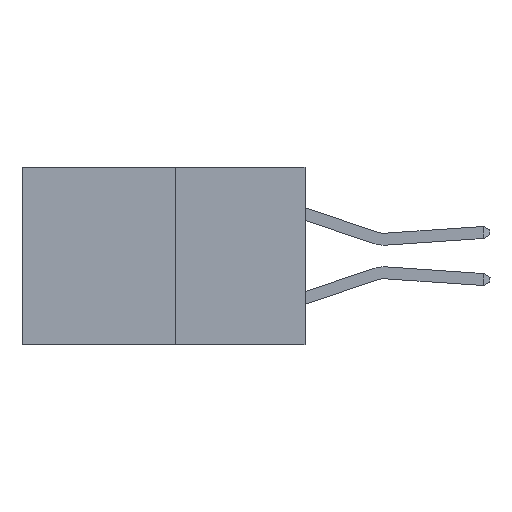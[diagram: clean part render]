
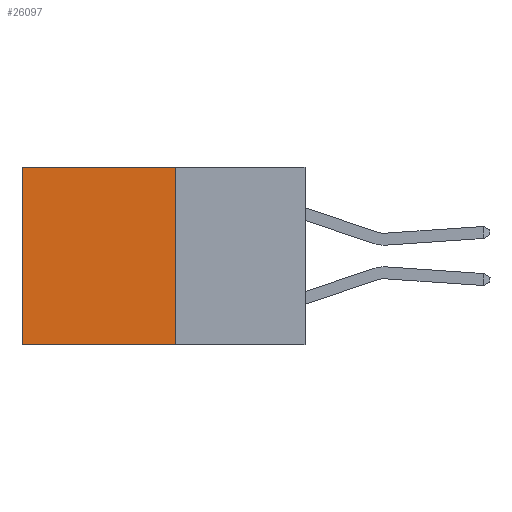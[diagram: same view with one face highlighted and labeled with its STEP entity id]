
A CAD part, left-side view. The second image highlights one B-rep face of the part: STEP entity #26097.
In plain terms, the highlighted planar face has unit normal (-1, 0, 0).
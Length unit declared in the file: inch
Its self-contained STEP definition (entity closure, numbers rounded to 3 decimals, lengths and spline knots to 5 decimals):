
#1031 = ORIENTED_EDGE ( 'NONE', *, *, #2963, .T. ) ;
#2616 = LINE ( 'NONE', #23293, #19332 ) ;
#2730 = LINE ( 'NONE', #22361, #3410 ) ;
#2963 = EDGE_CURVE ( 'NONE', #20592, #20436, #19629, .T. ) ;
#3410 = VECTOR ( 'NONE', #9292, 39.37008 ) ;
#3636 = VERTEX_POINT ( 'NONE', #18526 ) ;
#3870 = ORIENTED_EDGE ( 'NONE', *, *, #28075, .T. ) ;
#4586 = ORIENTED_EDGE ( 'NONE', *, *, #19576, .F. ) ;
#6217 = DIRECTION ( 'NONE',  ( 1., 0., 0. ) ) ;
#6589 = ORIENTED_EDGE ( 'NONE', *, *, #9121, .F. ) ;
#6935 = VERTEX_POINT ( 'NONE', #13581 ) ;
#7030 = VECTOR ( 'NONE', #12642, 39.37008 ) ;
#8045 = DIRECTION ( 'NONE',  ( 0., 1., 0. ) ) ;
#9121 = EDGE_CURVE ( 'NONE', #6935, #3636, #2616, .T. ) ;
#9292 = DIRECTION ( 'NONE',  ( 0., 0., -1. ) ) ;
#10042 = AXIS2_PLACEMENT_3D ( 'NONE', #19302, #6217, #21448 ) ;
#11551 = CARTESIAN_POINT ( 'NONE',  ( 0.277, 0.27, 0. ) ) ;
#12642 = DIRECTION ( 'NONE',  ( 0., 0., -1. ) ) ;
#13136 = VECTOR ( 'NONE', #20878, 39.37008 ) ;
#13581 = CARTESIAN_POINT ( 'NONE',  ( 0.277, 0.27, -0.37 ) ) ;
#13749 = EDGE_LOOP ( 'NONE', ( #3870, #6589, #4586, #1031 ) ) ;
#14979 = CARTESIAN_POINT ( 'NONE',  ( 0.277, 0.27, 0. ) ) ;
#18526 = CARTESIAN_POINT ( 'NONE',  ( 0.277, 0.59, -0.37 ) ) ;
#18654 = LINE ( 'NONE', #27818, #7030 ) ;
#19302 = CARTESIAN_POINT ( 'NONE',  ( 0.277, 0.27, -0.37 ) ) ;
#19332 = VECTOR ( 'NONE', #8045, 39.37008 ) ;
#19576 = EDGE_CURVE ( 'NONE', #20592, #6935, #18654, .T. ) ;
#19629 = LINE ( 'NONE', #14979, #13136 ) ;
#20436 = VERTEX_POINT ( 'NONE', #21819 ) ;
#20592 = VERTEX_POINT ( 'NONE', #11551 ) ;
#20878 = DIRECTION ( 'NONE',  ( 0., 1., 0. ) ) ;
#21448 = DIRECTION ( 'NONE',  ( 0., 0., -1. ) ) ;
#21819 = CARTESIAN_POINT ( 'NONE',  ( 0.277, 0.59, 0. ) ) ;
#22361 = CARTESIAN_POINT ( 'NONE',  ( 0.277, 0.59, -0.37 ) ) ;
#23293 = CARTESIAN_POINT ( 'NONE',  ( 0.277, 0.27, -0.37 ) ) ;
#25848 = FACE_OUTER_BOUND ( 'NONE', #13749, .T. ) ;
#26097 = ADVANCED_FACE ( 'NONE', ( #25848 ), #27874, .F. ) ;
#27818 = CARTESIAN_POINT ( 'NONE',  ( 0.277, 0.27, -0.37 ) ) ;
#27874 = PLANE ( 'NONE',  #10042 ) ;
#28075 = EDGE_CURVE ( 'NONE', #20436, #3636, #2730, .T. ) ;
